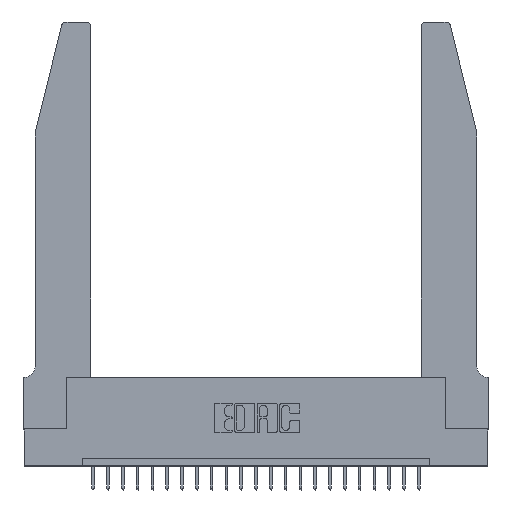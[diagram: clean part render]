
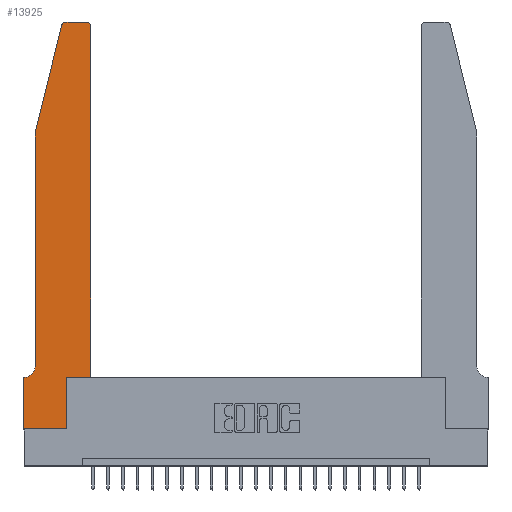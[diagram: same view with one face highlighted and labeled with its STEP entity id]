
A CAD part, top view. The second image highlights one B-rep face of the part: STEP entity #13925.
In plain terms, the highlighted planar face has unit normal (0, 0, 1).
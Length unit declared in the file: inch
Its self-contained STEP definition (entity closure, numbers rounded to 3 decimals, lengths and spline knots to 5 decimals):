
#136 = CARTESIAN_POINT ( 'NONE',  ( 0.2865, 0., 0.37 ) ) ;
#233 = DIRECTION ( 'NONE',  ( 0., -1., 0. ) ) ;
#290 = DIRECTION ( 'NONE',  ( 0., 0., 1. ) ) ;
#606 = VERTEX_POINT ( 'NONE', #1054 ) ;
#767 = VECTOR ( 'NONE', #19597, 39.37008 ) ;
#939 = DIRECTION ( 'NONE',  ( -0.239, -0.971, 0. ) ) ;
#1054 = CARTESIAN_POINT ( 'NONE',  ( 0.2865, 0.35, 0.37 ) ) ;
#1121 = ORIENTED_EDGE ( 'NONE', *, *, #9525, .T. ) ;
#1361 = EDGE_CURVE ( 'NONE', #19891, #4105, #11052, .T. ) ;
#1625 = CARTESIAN_POINT ( 'NONE',  ( 0.0755, 0.35, 0.37 ) ) ;
#2009 = DIRECTION ( 'NONE',  ( 1., 0., 0. ) ) ;
#2427 = VECTOR ( 'NONE', #233, 39.37008 ) ;
#2701 = CARTESIAN_POINT ( 'NONE',  ( 0.284, 2.72, 0.37 ) ) ;
#2773 = CARTESIAN_POINT ( 'NONE',  ( 0.0755, 0.42, 0.37 ) ) ;
#2857 = CIRCLE ( 'NONE', #15966, 0.03 ) ;
#2980 = EDGE_CURVE ( 'NONE', #7018, #3684, #3178, .T. ) ;
#3178 = LINE ( 'NONE', #15457, #10955 ) ;
#3446 = FACE_OUTER_BOUND ( 'NONE', #19572, .T. ) ;
#3455 = AXIS2_PLACEMENT_3D ( 'NONE', #3597, #11365, #15207 ) ;
#3533 = ORIENTED_EDGE ( 'NONE', *, *, #13938, .T. ) ;
#3597 = CARTESIAN_POINT ( 'NONE',  ( 0.0055, 0.42, 0.37 ) ) ;
#3684 = VERTEX_POINT ( 'NONE', #16989 ) ;
#4105 = VERTEX_POINT ( 'NONE', #12787 ) ;
#4357 = EDGE_CURVE ( 'NONE', #606, #23246, #14427, .T. ) ;
#4461 = CIRCLE ( 'NONE', #18450, 0.03 ) ;
#4675 = VERTEX_POINT ( 'NONE', #136 ) ;
#5129 = EDGE_CURVE ( 'NONE', #20590, #19891, #11693, .T. ) ;
#5425 = PLANE ( 'NONE',  #8830 ) ;
#5927 = LINE ( 'NONE', #1625, #19879 ) ;
#6116 = VECTOR ( 'NONE', #10839, 39.37008 ) ;
#6331 = ORIENTED_EDGE ( 'NONE', *, *, #7026, .T. ) ;
#6452 = EDGE_CURVE ( 'NONE', #21881, #12525, #4461, .T. ) ;
#6567 = VECTOR ( 'NONE', #939, 39.37008 ) ;
#6599 = VERTEX_POINT ( 'NONE', #14526 ) ;
#6732 = LINE ( 'NONE', #9597, #21901 ) ;
#7018 = VERTEX_POINT ( 'NONE', #7141 ) ;
#7026 = EDGE_CURVE ( 'NONE', #4105, #7018, #5927, .T. ) ;
#7141 = CARTESIAN_POINT ( 'NONE',  ( 0., 0.35, 0.37 ) ) ;
#7154 = LINE ( 'NONE', #19957, #6567 ) ;
#8733 = DIRECTION ( 'NONE',  ( 1., 0., 0. ) ) ;
#8830 = AXIS2_PLACEMENT_3D ( 'NONE', #11419, #16692, #8733 ) ;
#8949 = EDGE_CURVE ( 'NONE', #23246, #21881, #10908, .T. ) ;
#9525 = EDGE_CURVE ( 'NONE', #12525, #13986, #24319, .T. ) ;
#9597 = CARTESIAN_POINT ( 'NONE',  ( 0., 0., 0.37 ) ) ;
#10839 = DIRECTION ( 'NONE',  ( 0., 1., 0. ) ) ;
#10908 = LINE ( 'NONE', #24367, #6116 ) ;
#10955 = VECTOR ( 'NONE', #11618, 39.37008 ) ;
#11052 = CIRCLE ( 'NONE', #3455, 0.07 ) ;
#11365 = DIRECTION ( 'NONE',  ( 0., 0., -1. ) ) ;
#11419 = CARTESIAN_POINT ( 'NONE',  ( 0., 0.35, 0.37 ) ) ;
#11618 = DIRECTION ( 'NONE',  ( 0., -1., 0. ) ) ;
#11644 = DIRECTION ( 'NONE',  ( 1., 0., 0. ) ) ;
#11693 = LINE ( 'NONE', #20369, #2427 ) ;
#11737 = EDGE_CURVE ( 'NONE', #6599, #20590, #7154, .T. ) ;
#12525 = VERTEX_POINT ( 'NONE', #18791 ) ;
#12718 = CARTESIAN_POINT ( 'NONE',  ( 0.4505, 2.72, 0.37 ) ) ;
#12787 = CARTESIAN_POINT ( 'NONE',  ( 0.0055, 0.35, 0.37 ) ) ;
#13493 = DIRECTION ( 'NONE',  ( 1., 0., 0. ) ) ;
#13805 = ORIENTED_EDGE ( 'NONE', *, *, #4357, .T. ) ;
#13862 = CARTESIAN_POINT ( 'NONE',  ( 0.2605, 2.75, 0.37 ) ) ;
#13925 = ADVANCED_FACE ( 'NONE', ( #3446 ), #5425, .T. ) ;
#13938 = EDGE_CURVE ( 'NONE', #13986, #6599, #2857, .T. ) ;
#13986 = VERTEX_POINT ( 'NONE', #21170 ) ;
#14427 = LINE ( 'NONE', #20729, #20974 ) ;
#14526 = CARTESIAN_POINT ( 'NONE',  ( 0.25487, 2.72718, 0.37 ) ) ;
#15207 = DIRECTION ( 'NONE',  ( -1., 0., 0. ) ) ;
#15213 = CARTESIAN_POINT ( 'NONE',  ( 0.2865, 0.35, 0.37 ) ) ;
#15437 = ORIENTED_EDGE ( 'NONE', *, *, #1361, .T. ) ;
#15457 = CARTESIAN_POINT ( 'NONE',  ( 0., 0., 0.37 ) ) ;
#15796 = CARTESIAN_POINT ( 'NONE',  ( 0.0755, 2., 0.37 ) ) ;
#15966 = AXIS2_PLACEMENT_3D ( 'NONE', #2701, #290, #11644 ) ;
#16090 = DIRECTION ( 'NONE',  ( 1., 0., 0. ) ) ;
#16332 = ORIENTED_EDGE ( 'NONE', *, *, #11737, .T. ) ;
#16692 = DIRECTION ( 'NONE',  ( 0., 0., 1. ) ) ;
#16989 = CARTESIAN_POINT ( 'NONE',  ( 0., 0., 0.37 ) ) ;
#17249 = LINE ( 'NONE', #15213, #18735 ) ;
#17872 = DIRECTION ( 'NONE',  ( 0., 0., 1. ) ) ;
#18022 = ORIENTED_EDGE ( 'NONE', *, *, #18480, .T. ) ;
#18450 = AXIS2_PLACEMENT_3D ( 'NONE', #23898, #17872, #16090 ) ;
#18480 = EDGE_CURVE ( 'NONE', #3684, #4675, #6732, .T. ) ;
#18522 = ORIENTED_EDGE ( 'NONE', *, *, #8949, .T. ) ;
#18735 = VECTOR ( 'NONE', #21158, 39.37008 ) ;
#18751 = ORIENTED_EDGE ( 'NONE', *, *, #5129, .T. ) ;
#18791 = CARTESIAN_POINT ( 'NONE',  ( 0.4205, 2.75, 0.37 ) ) ;
#18955 = ORIENTED_EDGE ( 'NONE', *, *, #2980, .T. ) ;
#19186 = CARTESIAN_POINT ( 'NONE',  ( 0.4505, 0.35, 0.37 ) ) ;
#19572 = EDGE_LOOP ( 'NONE', ( #1121, #3533, #16332, #18751, #15437, #6331, #18955, #18022, #23344, #13805, #18522, #22596 ) ) ;
#19597 = DIRECTION ( 'NONE',  ( -1., 0., 0. ) ) ;
#19879 = VECTOR ( 'NONE', #20663, 39.37008 ) ;
#19891 = VERTEX_POINT ( 'NONE', #2773 ) ;
#19957 = CARTESIAN_POINT ( 'NONE',  ( 0.0755, 2., 0.37 ) ) ;
#20369 = CARTESIAN_POINT ( 'NONE',  ( 0.0755, 2., 0.37 ) ) ;
#20590 = VERTEX_POINT ( 'NONE', #15796 ) ;
#20663 = DIRECTION ( 'NONE',  ( -1., 0., 0. ) ) ;
#20729 = CARTESIAN_POINT ( 'NONE',  ( 0.4505, 0.35, 0.37 ) ) ;
#20974 = VECTOR ( 'NONE', #13493, 39.37008 ) ;
#21158 = DIRECTION ( 'NONE',  ( 0., 1., 0. ) ) ;
#21170 = CARTESIAN_POINT ( 'NONE',  ( 0.284, 2.75, 0.37 ) ) ;
#21881 = VERTEX_POINT ( 'NONE', #12718 ) ;
#21901 = VECTOR ( 'NONE', #2009, 39.37008 ) ;
#22144 = EDGE_CURVE ( 'NONE', #4675, #606, #17249, .T. ) ;
#22596 = ORIENTED_EDGE ( 'NONE', *, *, #6452, .T. ) ;
#23246 = VERTEX_POINT ( 'NONE', #19186 ) ;
#23344 = ORIENTED_EDGE ( 'NONE', *, *, #22144, .T. ) ;
#23898 = CARTESIAN_POINT ( 'NONE',  ( 0.4205, 2.72, 0.37 ) ) ;
#24319 = LINE ( 'NONE', #13862, #767 ) ;
#24367 = CARTESIAN_POINT ( 'NONE',  ( 0.4505, 0.35, 0.37 ) ) ;
